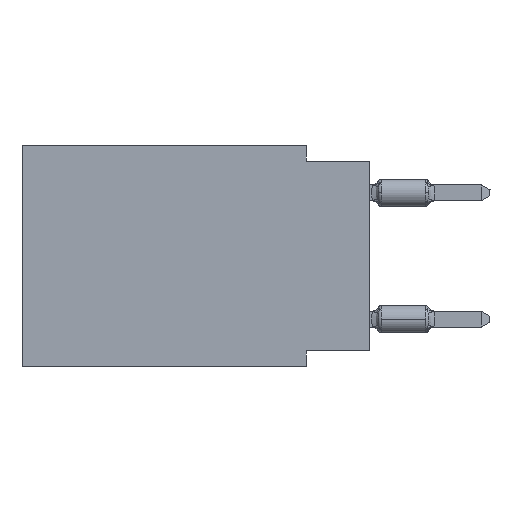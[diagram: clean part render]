
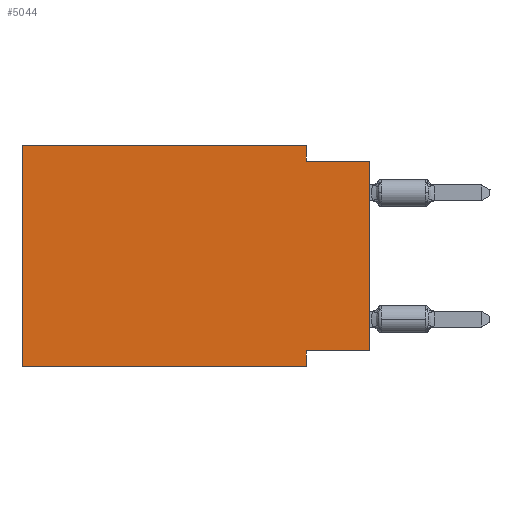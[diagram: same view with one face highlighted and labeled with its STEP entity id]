
A CAD part, left-side view. The second image highlights one B-rep face of the part: STEP entity #5044.
In plain terms, the highlighted planar face has unit normal (-1, 0, 0).
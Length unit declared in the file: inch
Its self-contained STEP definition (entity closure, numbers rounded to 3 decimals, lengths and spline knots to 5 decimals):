
#447 = DIRECTION ( 'NONE',  ( 0., 0., -1. ) ) ;
#771 = LINE ( 'NONE', #8753, #1510 ) ;
#1510 = VECTOR ( 'NONE', #21837, 39.37008 ) ;
#1818 = EDGE_CURVE ( 'NONE', #2674, #23076, #24314, .T. ) ;
#2597 = VECTOR ( 'NONE', #447, 39.37008 ) ;
#2674 = VERTEX_POINT ( 'NONE', #18643 ) ;
#3335 = DIRECTION ( 'NONE',  ( 1., 0., 0. ) ) ;
#3351 = VERTEX_POINT ( 'NONE', #14084 ) ;
#3680 = ORIENTED_EDGE ( 'NONE', *, *, #10910, .F. ) ;
#4290 = LINE ( 'NONE', #22219, #22063 ) ;
#5044 = ADVANCED_FACE ( 'NONE', ( #24568 ), #6668, .F. ) ;
#5063 = LINE ( 'NONE', #9982, #11169 ) ;
#6194 = DIRECTION ( 'NONE',  ( 0., -1., 0. ) ) ;
#6668 = PLANE ( 'NONE',  #14834 ) ;
#6722 = LINE ( 'NONE', #8424, #2597 ) ;
#6809 = VERTEX_POINT ( 'NONE', #25295 ) ;
#6879 = CARTESIAN_POINT ( 'NONE',  ( 0., 0.55, 0. ) ) ;
#7854 = VERTEX_POINT ( 'NONE', #6879 ) ;
#7903 = CARTESIAN_POINT ( 'NONE',  ( 0., 0.55, 0. ) ) ;
#8021 = EDGE_CURVE ( 'NONE', #7854, #2674, #8032, .T. ) ;
#8032 = LINE ( 'NONE', #7903, #17613 ) ;
#8196 = EDGE_CURVE ( 'NONE', #3351, #16067, #6722, .T. ) ;
#8424 = CARTESIAN_POINT ( 'NONE',  ( 0., 0.1, -0.35 ) ) ;
#8753 = CARTESIAN_POINT ( 'NONE',  ( 0., 0.55, -0.35 ) ) ;
#8774 = CARTESIAN_POINT ( 'NONE',  ( 0., 0., -0.325 ) ) ;
#9773 = DIRECTION ( 'NONE',  ( 0., 1., 0. ) ) ;
#9982 = CARTESIAN_POINT ( 'NONE',  ( 0., 0., -0.025 ) ) ;
#10298 = VERTEX_POINT ( 'NONE', #21292 ) ;
#10910 = EDGE_CURVE ( 'NONE', #6809, #7854, #24735, .T. ) ;
#11169 = VECTOR ( 'NONE', #21510, 39.37008 ) ;
#11904 = VERTEX_POINT ( 'NONE', #8774 ) ;
#12468 = VECTOR ( 'NONE', #20957, 39.37008 ) ;
#13186 = EDGE_LOOP ( 'NONE', ( #20921, #14895, #25224, #23942, #3680, #23141, #17528, #18049 ) ) ;
#13258 = DIRECTION ( 'NONE',  ( 0., 0., -1. ) ) ;
#14084 = CARTESIAN_POINT ( 'NONE',  ( 0., 0.1, -0.325 ) ) ;
#14372 = CARTESIAN_POINT ( 'NONE',  ( 0., 0.1, 0. ) ) ;
#14834 = AXIS2_PLACEMENT_3D ( 'NONE', #19053, #3335, #13258 ) ;
#14895 = ORIENTED_EDGE ( 'NONE', *, *, #21673, .F. ) ;
#15073 = EDGE_CURVE ( 'NONE', #11904, #3351, #16191, .T. ) ;
#15359 = CARTESIAN_POINT ( 'NONE',  ( 0., 0.1, -0.35 ) ) ;
#15945 = CARTESIAN_POINT ( 'NONE',  ( 0., 0., -0.325 ) ) ;
#15974 = DIRECTION ( 'NONE',  ( 0., 0., -1. ) ) ;
#16067 = VERTEX_POINT ( 'NONE', #15359 ) ;
#16191 = LINE ( 'NONE', #15945, #23424 ) ;
#17528 = ORIENTED_EDGE ( 'NONE', *, *, #8196, .F. ) ;
#17577 = VECTOR ( 'NONE', #15974, 39.37008 ) ;
#17613 = VECTOR ( 'NONE', #6194, 39.37008 ) ;
#18049 = ORIENTED_EDGE ( 'NONE', *, *, #15073, .F. ) ;
#18602 = EDGE_CURVE ( 'NONE', #6809, #16067, #771, .T. ) ;
#18643 = CARTESIAN_POINT ( 'NONE',  ( 0., 0.1, 0. ) ) ;
#19053 = CARTESIAN_POINT ( 'NONE',  ( 0., 0.55, 0. ) ) ;
#20921 = ORIENTED_EDGE ( 'NONE', *, *, #21430, .T. ) ;
#20957 = DIRECTION ( 'NONE',  ( 0., 0., 1. ) ) ;
#21292 = CARTESIAN_POINT ( 'NONE',  ( 0., 0., -0.025 ) ) ;
#21430 = EDGE_CURVE ( 'NONE', #11904, #10298, #4290, .T. ) ;
#21510 = DIRECTION ( 'NONE',  ( 0., -1., 0. ) ) ;
#21673 = EDGE_CURVE ( 'NONE', #23076, #10298, #5063, .T. ) ;
#21837 = DIRECTION ( 'NONE',  ( 0., -1., 0. ) ) ;
#22063 = VECTOR ( 'NONE', #22342, 39.37008 ) ;
#22219 = CARTESIAN_POINT ( 'NONE',  ( 0., 0., 0. ) ) ;
#22342 = DIRECTION ( 'NONE',  ( 0., 0., 1. ) ) ;
#22385 = CARTESIAN_POINT ( 'NONE',  ( 0., 0.55, 0. ) ) ;
#22916 = CARTESIAN_POINT ( 'NONE',  ( 0., 0.1, -0.025 ) ) ;
#23076 = VERTEX_POINT ( 'NONE', #22916 ) ;
#23141 = ORIENTED_EDGE ( 'NONE', *, *, #18602, .T. ) ;
#23424 = VECTOR ( 'NONE', #9773, 39.37008 ) ;
#23942 = ORIENTED_EDGE ( 'NONE', *, *, #8021, .F. ) ;
#24314 = LINE ( 'NONE', #14372, #17577 ) ;
#24568 = FACE_OUTER_BOUND ( 'NONE', #13186, .T. ) ;
#24735 = LINE ( 'NONE', #22385, #12468 ) ;
#25224 = ORIENTED_EDGE ( 'NONE', *, *, #1818, .F. ) ;
#25295 = CARTESIAN_POINT ( 'NONE',  ( 0., 0.55, -0.35 ) ) ;
